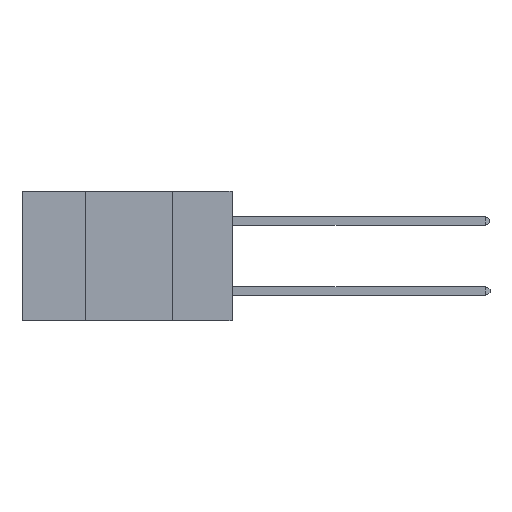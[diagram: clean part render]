
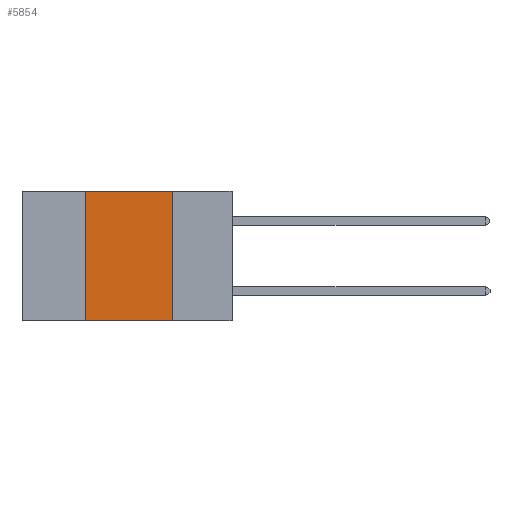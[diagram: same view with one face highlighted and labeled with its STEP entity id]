
A CAD part, left-side view. The second image highlights one B-rep face of the part: STEP entity #5854.
In plain terms, the highlighted planar face has unit normal (-1, 0, 0).
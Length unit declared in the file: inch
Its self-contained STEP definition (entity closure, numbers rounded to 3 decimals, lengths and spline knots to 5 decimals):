
#573 = LINE ( 'NONE', #12714, #8571 ) ;
#1143 = VECTOR ( 'NONE', #9443, 39.37008 ) ;
#1865 = ORIENTED_EDGE ( 'NONE', *, *, #22343, .F. ) ;
#3357 = VERTEX_POINT ( 'NONE', #3661 ) ;
#3661 = CARTESIAN_POINT ( 'NONE',  ( 0., 0.17, 0. ) ) ;
#5854 = ADVANCED_FACE ( 'NONE', ( #17425 ), #13190, .F. ) ;
#6452 = CARTESIAN_POINT ( 'NONE',  ( 0., 0.17, -0.37 ) ) ;
#6536 = VERTEX_POINT ( 'NONE', #15224 ) ;
#7952 = CARTESIAN_POINT ( 'NONE',  ( 0., 0.6, 0. ) ) ;
#8571 = VECTOR ( 'NONE', #18021, 39.37008 ) ;
#8928 = ORIENTED_EDGE ( 'NONE', *, *, #18928, .T. ) ;
#9443 = DIRECTION ( 'NONE',  ( 0., 0., 1. ) ) ;
#10102 = DIRECTION ( 'NONE',  ( 0., 0., -1. ) ) ;
#10267 = LINE ( 'NONE', #21818, #14741 ) ;
#11824 = ORIENTED_EDGE ( 'NONE', *, *, #18743, .F. ) ;
#11872 = VERTEX_POINT ( 'NONE', #21281 ) ;
#11890 = LINE ( 'NONE', #22555, #16629 ) ;
#12390 = LINE ( 'NONE', #18648, #1143 ) ;
#12714 = CARTESIAN_POINT ( 'NONE',  ( 0., 0.6, 0. ) ) ;
#13190 = PLANE ( 'NONE',  #20817 ) ;
#13418 = DIRECTION ( 'NONE',  ( 0., 0., -1. ) ) ;
#14741 = VECTOR ( 'NONE', #20108, 39.37008 ) ;
#15224 = CARTESIAN_POINT ( 'NONE',  ( 0., 0.42, 0. ) ) ;
#15603 = EDGE_CURVE ( 'NONE', #6536, #3357, #573, .T. ) ;
#16462 = VERTEX_POINT ( 'NONE', #6452 ) ;
#16629 = VECTOR ( 'NONE', #13418, 39.37008 ) ;
#17425 = FACE_OUTER_BOUND ( 'NONE', #17988, .T. ) ;
#17632 = DIRECTION ( 'NONE',  ( 1., 0., 0. ) ) ;
#17988 = EDGE_LOOP ( 'NONE', ( #1865, #19911, #11824, #8928 ) ) ;
#18021 = DIRECTION ( 'NONE',  ( 0., -1., 0. ) ) ;
#18648 = CARTESIAN_POINT ( 'NONE',  ( 0., 0.42, 0. ) ) ;
#18743 = EDGE_CURVE ( 'NONE', #11872, #6536, #12390, .T. ) ;
#18928 = EDGE_CURVE ( 'NONE', #11872, #16462, #10267, .T. ) ;
#19911 = ORIENTED_EDGE ( 'NONE', *, *, #15603, .F. ) ;
#20108 = DIRECTION ( 'NONE',  ( 0., -1., 0. ) ) ;
#20817 = AXIS2_PLACEMENT_3D ( 'NONE', #7952, #17632, #10102 ) ;
#21281 = CARTESIAN_POINT ( 'NONE',  ( 0., 0.42, -0.37 ) ) ;
#21818 = CARTESIAN_POINT ( 'NONE',  ( 0., 0.6, -0.37 ) ) ;
#22343 = EDGE_CURVE ( 'NONE', #3357, #16462, #11890, .T. ) ;
#22555 = CARTESIAN_POINT ( 'NONE',  ( 0., 0.17, 0. ) ) ;
